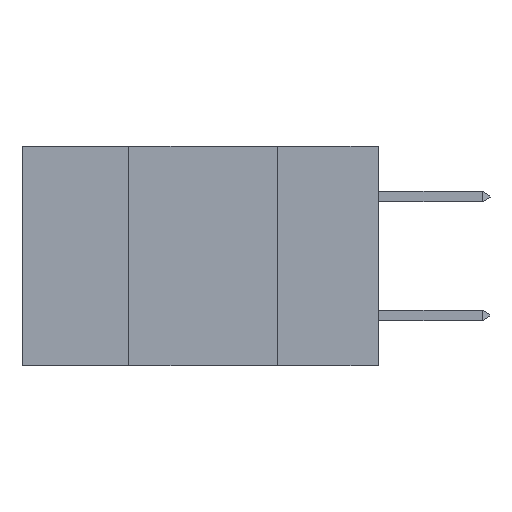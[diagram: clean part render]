
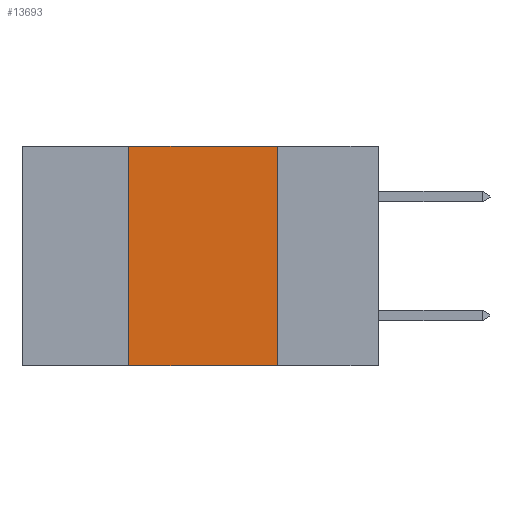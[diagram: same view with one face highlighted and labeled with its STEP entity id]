
A CAD part, left-side view. The second image highlights one B-rep face of the part: STEP entity #13693.
In plain terms, the highlighted planar face has unit normal (-1, 0, 0).
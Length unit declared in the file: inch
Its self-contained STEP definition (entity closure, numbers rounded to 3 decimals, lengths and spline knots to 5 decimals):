
#2026 = VECTOR ( 'NONE', #30339, 39.37008 ) ;
#3375 = DIRECTION ( 'NONE',  ( 1., 0., 0. ) ) ;
#4648 = DIRECTION ( 'NONE',  ( 0., 0., -1. ) ) ;
#5485 = VECTOR ( 'NONE', #4648, 39.37008 ) ;
#6465 = DIRECTION ( 'NONE',  ( 0., -1., 0. ) ) ;
#6609 = EDGE_CURVE ( 'NONE', #29550, #17535, #24458, .T. ) ;
#8265 = CARTESIAN_POINT ( 'NONE',  ( 0., 0.42, -0.37 ) ) ;
#8560 = FACE_OUTER_BOUND ( 'NONE', #20502, .T. ) ;
#8638 = EDGE_CURVE ( 'NONE', #16729, #16203, #23230, .T. ) ;
#8654 = DIRECTION ( 'NONE',  ( 0., -1., 0. ) ) ;
#9466 = VECTOR ( 'NONE', #8654, 39.37008 ) ;
#9755 = EDGE_CURVE ( 'NONE', #16729, #17535, #14306, .T. ) ;
#10631 = PLANE ( 'NONE',  #22209 ) ;
#10805 = ORIENTED_EDGE ( 'NONE', *, *, #9755, .T. ) ;
#11035 = ORIENTED_EDGE ( 'NONE', *, *, #8638, .F. ) ;
#12138 = LINE ( 'NONE', #26994, #24047 ) ;
#13693 = ADVANCED_FACE ( 'NONE', ( #8560 ), #10631, .F. ) ;
#14038 = ORIENTED_EDGE ( 'NONE', *, *, #28456, .F. ) ;
#14306 = LINE ( 'NONE', #15436, #9466 ) ;
#15436 = CARTESIAN_POINT ( 'NONE',  ( 0., 0.6, -0.37 ) ) ;
#16203 = VERTEX_POINT ( 'NONE', #29869 ) ;
#16729 = VERTEX_POINT ( 'NONE', #8265 ) ;
#17121 = CARTESIAN_POINT ( 'NONE',  ( 0., 0.17, 0. ) ) ;
#17535 = VERTEX_POINT ( 'NONE', #27619 ) ;
#20502 = EDGE_LOOP ( 'NONE', ( #23194, #14038, #11035, #10805 ) ) ;
#22209 = AXIS2_PLACEMENT_3D ( 'NONE', #27529, #3375, #27110 ) ;
#23194 = ORIENTED_EDGE ( 'NONE', *, *, #6609, .F. ) ;
#23230 = LINE ( 'NONE', #23392, #2026 ) ;
#23392 = CARTESIAN_POINT ( 'NONE',  ( 0., 0.42, 0. ) ) ;
#24047 = VECTOR ( 'NONE', #6465, 39.37008 ) ;
#24458 = LINE ( 'NONE', #29021, #5485 ) ;
#26994 = CARTESIAN_POINT ( 'NONE',  ( 0., 0.6, 0. ) ) ;
#27110 = DIRECTION ( 'NONE',  ( 0., 0., -1. ) ) ;
#27529 = CARTESIAN_POINT ( 'NONE',  ( 0., 0.6, 0. ) ) ;
#27619 = CARTESIAN_POINT ( 'NONE',  ( 0., 0.17, -0.37 ) ) ;
#28456 = EDGE_CURVE ( 'NONE', #16203, #29550, #12138, .T. ) ;
#29021 = CARTESIAN_POINT ( 'NONE',  ( 0., 0.17, 0. ) ) ;
#29550 = VERTEX_POINT ( 'NONE', #17121 ) ;
#29869 = CARTESIAN_POINT ( 'NONE',  ( 0., 0.42, 0. ) ) ;
#30339 = DIRECTION ( 'NONE',  ( 0., 0., 1. ) ) ;
